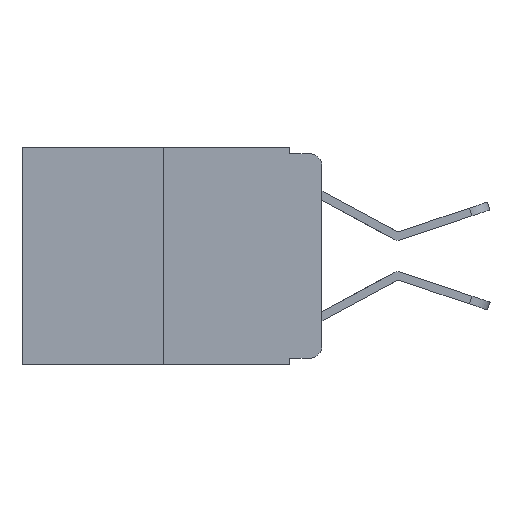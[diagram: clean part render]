
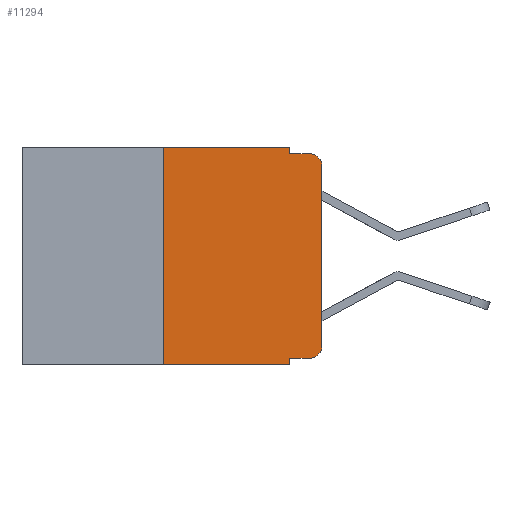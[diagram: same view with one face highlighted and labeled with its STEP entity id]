
A CAD part, left-side view. The second image highlights one B-rep face of the part: STEP entity #11294.
In plain terms, the highlighted planar face has unit normal (-1, 0, 0).
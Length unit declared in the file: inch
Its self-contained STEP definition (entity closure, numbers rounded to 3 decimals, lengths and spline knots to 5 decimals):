
#232 = ORIENTED_EDGE ( 'NONE', *, *, #2204, .T. ) ;
#239 = VERTEX_POINT ( 'NONE', #2413 ) ;
#660 = CARTESIAN_POINT ( 'NONE',  ( 0., 0.051, -0.333 ) ) ;
#976 = LINE ( 'NONE', #1374, #8656 ) ;
#1017 = ORIENTED_EDGE ( 'NONE', *, *, #7707, .T. ) ;
#1066 = LINE ( 'NONE', #2207, #6061 ) ;
#1285 = DIRECTION ( 'NONE',  ( 0., -1., 0. ) ) ;
#1374 = CARTESIAN_POINT ( 'NONE',  ( 0., 0.051, 0. ) ) ;
#1390 = VERTEX_POINT ( 'NONE', #2370 ) ;
#1683 = PLANE ( 'NONE',  #5880 ) ;
#1869 = ORIENTED_EDGE ( 'NONE', *, *, #4636, .F. ) ;
#2021 = ORIENTED_EDGE ( 'NONE', *, *, #11806, .T. ) ;
#2199 = ORIENTED_EDGE ( 'NONE', *, *, #2746, .F. ) ;
#2204 = EDGE_CURVE ( 'NONE', #7102, #12849, #12438, .T. ) ;
#2207 = CARTESIAN_POINT ( 'NONE',  ( 0., 0.051, 0. ) ) ;
#2220 = VECTOR ( 'NONE', #12950, 39.37008 ) ;
#2251 = CARTESIAN_POINT ( 'NONE',  ( 0., 0.051, 0. ) ) ;
#2370 = CARTESIAN_POINT ( 'NONE',  ( 0., 0.25, -0.343 ) ) ;
#2413 = CARTESIAN_POINT ( 'NONE',  ( 0., 0., -0.03 ) ) ;
#2540 = DIRECTION ( 'NONE',  ( 0., 0., 1. ) ) ;
#2746 = EDGE_CURVE ( 'NONE', #10735, #5289, #976, .T. ) ;
#2845 = VECTOR ( 'NONE', #2850, 39.37008 ) ;
#2850 = DIRECTION ( 'NONE',  ( 0., -1., 0. ) ) ;
#3039 = AXIS2_PLACEMENT_3D ( 'NONE', #7736, #11798, #8717 ) ;
#3389 = DIRECTION ( 'NONE',  ( -1., 0., 0. ) ) ;
#3440 = EDGE_CURVE ( 'NONE', #5174, #10951, #9250, .T. ) ;
#3813 = VERTEX_POINT ( 'NONE', #8427 ) ;
#3839 = DIRECTION ( 'NONE',  ( 0., 0., -1. ) ) ;
#4157 = AXIS2_PLACEMENT_3D ( 'NONE', #6249, #3389, #8303 ) ;
#4255 = DIRECTION ( 'NONE',  ( 0., -1., 0. ) ) ;
#4365 = ORIENTED_EDGE ( 'NONE', *, *, #9212, .F. ) ;
#4636 = EDGE_CURVE ( 'NONE', #3813, #7474, #8754, .T. ) ;
#5139 = CARTESIAN_POINT ( 'NONE',  ( 0., 0.25, 0. ) ) ;
#5174 = VERTEX_POINT ( 'NONE', #5139 ) ;
#5289 = VERTEX_POINT ( 'NONE', #11587 ) ;
#5491 = LINE ( 'NONE', #6054, #9580 ) ;
#5695 = ORIENTED_EDGE ( 'NONE', *, *, #3440, .F. ) ;
#5764 = FACE_OUTER_BOUND ( 'NONE', #5803, .T. ) ;
#5803 = EDGE_LOOP ( 'NONE', ( #2021, #1017, #1869, #6306, #5695, #4365, #8126, #2199, #5906, #232 ) ) ;
#5880 = AXIS2_PLACEMENT_3D ( 'NONE', #8819, #9782, #3839 ) ;
#5906 = ORIENTED_EDGE ( 'NONE', *, *, #9051, .T. ) ;
#6054 = CARTESIAN_POINT ( 'NONE',  ( 0., 0.25, 0. ) ) ;
#6061 = VECTOR ( 'NONE', #9336, 39.37008 ) ;
#6165 = CARTESIAN_POINT ( 'NONE',  ( 0., 0.051, -0.01 ) ) ;
#6249 = CARTESIAN_POINT ( 'NONE',  ( 0., 0.02, -0.313 ) ) ;
#6306 = ORIENTED_EDGE ( 'NONE', *, *, #11926, .F. ) ;
#6590 = LINE ( 'NONE', #11885, #2220 ) ;
#6713 = CARTESIAN_POINT ( 'NONE',  ( 0., 0., -0.313 ) ) ;
#7003 = DIRECTION ( 'NONE',  ( 0., 0., 1. ) ) ;
#7102 = VERTEX_POINT ( 'NONE', #10293 ) ;
#7201 = CARTESIAN_POINT ( 'NONE',  ( 0., 0.02, -0.01 ) ) ;
#7474 = VERTEX_POINT ( 'NONE', #7201 ) ;
#7707 = EDGE_CURVE ( 'NONE', #239, #7474, #9289, .T. ) ;
#7736 = CARTESIAN_POINT ( 'NONE',  ( 0., 0.02, -0.03 ) ) ;
#8126 = ORIENTED_EDGE ( 'NONE', *, *, #8238, .T. ) ;
#8204 = CARTESIAN_POINT ( 'NONE',  ( 0., 0.473, -0.343 ) ) ;
#8238 = EDGE_CURVE ( 'NONE', #1390, #5289, #10232, .T. ) ;
#8303 = DIRECTION ( 'NONE',  ( 0., 0., -1. ) ) ;
#8427 = CARTESIAN_POINT ( 'NONE',  ( 0., 0.051, -0.01 ) ) ;
#8656 = VECTOR ( 'NONE', #10364, 39.37008 ) ;
#8659 = VECTOR ( 'NONE', #1285, 39.37008 ) ;
#8717 = DIRECTION ( 'NONE',  ( 0., 0., -1. ) ) ;
#8751 = VECTOR ( 'NONE', #2540, 39.37008 ) ;
#8754 = LINE ( 'NONE', #6165, #11432 ) ;
#8819 = CARTESIAN_POINT ( 'NONE',  ( 0., 0.473, 0. ) ) ;
#9051 = EDGE_CURVE ( 'NONE', #10735, #7102, #6590, .T. ) ;
#9212 = EDGE_CURVE ( 'NONE', #1390, #5174, #5491, .T. ) ;
#9250 = LINE ( 'NONE', #10944, #2845 ) ;
#9289 = CIRCLE ( 'NONE', #3039, 0.02 ) ;
#9336 = DIRECTION ( 'NONE',  ( 0., 0., -1. ) ) ;
#9580 = VECTOR ( 'NONE', #7003, 39.37008 ) ;
#9782 = DIRECTION ( 'NONE',  ( 1., 0., 0. ) ) ;
#10232 = LINE ( 'NONE', #8204, #8659 ) ;
#10293 = CARTESIAN_POINT ( 'NONE',  ( 0., 0.02, -0.333 ) ) ;
#10364 = DIRECTION ( 'NONE',  ( 0., 0., -1. ) ) ;
#10735 = VERTEX_POINT ( 'NONE', #660 ) ;
#10944 = CARTESIAN_POINT ( 'NONE',  ( 0., 0.473, 0. ) ) ;
#10951 = VERTEX_POINT ( 'NONE', #2251 ) ;
#11294 = ADVANCED_FACE ( 'NONE', ( #5764 ), #1683, .F. ) ;
#11432 = VECTOR ( 'NONE', #4255, 39.37008 ) ;
#11587 = CARTESIAN_POINT ( 'NONE',  ( 0., 0.051, -0.343 ) ) ;
#11666 = CARTESIAN_POINT ( 'NONE',  ( 0., 0., 0. ) ) ;
#11798 = DIRECTION ( 'NONE',  ( -1., 0., 0. ) ) ;
#11806 = EDGE_CURVE ( 'NONE', #12849, #239, #12384, .T. ) ;
#11885 = CARTESIAN_POINT ( 'NONE',  ( 0., 0.051, -0.333 ) ) ;
#11926 = EDGE_CURVE ( 'NONE', #10951, #3813, #1066, .T. ) ;
#12384 = LINE ( 'NONE', #11666, #8751 ) ;
#12438 = CIRCLE ( 'NONE', #4157, 0.02 ) ;
#12849 = VERTEX_POINT ( 'NONE', #6713 ) ;
#12950 = DIRECTION ( 'NONE',  ( 0., -1., 0. ) ) ;
